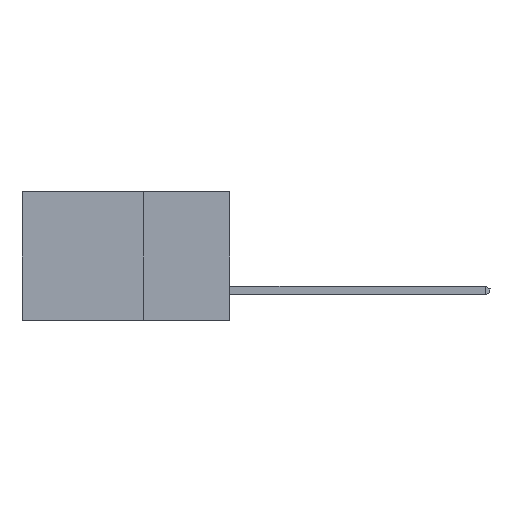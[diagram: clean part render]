
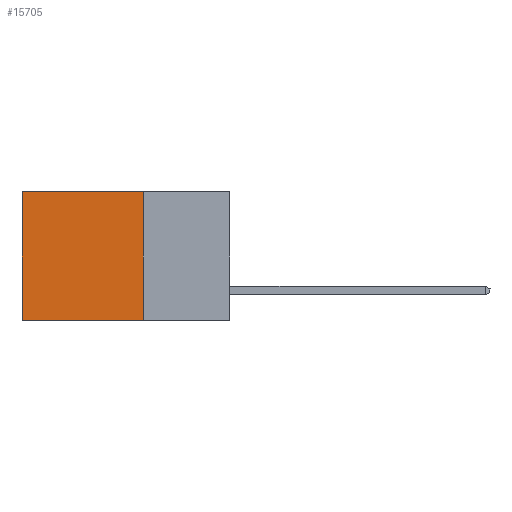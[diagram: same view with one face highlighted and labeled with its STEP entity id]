
A CAD part, left-side view. The second image highlights one B-rep face of the part: STEP entity #15705.
In plain terms, the highlighted planar face has unit normal (-1, 0, 0).
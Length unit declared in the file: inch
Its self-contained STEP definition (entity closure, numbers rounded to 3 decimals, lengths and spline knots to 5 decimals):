
#1093 = VERTEX_POINT ( 'NONE', #7252 ) ;
#1195 = DIRECTION ( 'NONE',  ( 0., 0., -1. ) ) ;
#1316 = ORIENTED_EDGE ( 'NONE', *, *, #8165, .T. ) ;
#1537 = AXIS2_PLACEMENT_3D ( 'NONE', #11090, #6801, #6607 ) ;
#2437 = ORIENTED_EDGE ( 'NONE', *, *, #10754, .F. ) ;
#2819 = EDGE_CURVE ( 'NONE', #3945, #1093, #11058, .T. ) ;
#3433 = LINE ( 'NONE', #9381, #17331 ) ;
#3897 = EDGE_LOOP ( 'NONE', ( #1316, #7428, #2437, #6747 ) ) ;
#3945 = VERTEX_POINT ( 'NONE', #3963 ) ;
#3952 = LINE ( 'NONE', #8041, #9803 ) ;
#3963 = CARTESIAN_POINT ( 'NONE',  ( 0.2615, 0.25, -0.37 ) ) ;
#5683 = CARTESIAN_POINT ( 'NONE',  ( 0.2615, 0.6, -0.37 ) ) ;
#6607 = DIRECTION ( 'NONE',  ( 0., 0., -1. ) ) ;
#6747 = ORIENTED_EDGE ( 'NONE', *, *, #13581, .T. ) ;
#6771 = DIRECTION ( 'NONE',  ( 0., 1., 0. ) ) ;
#6801 = DIRECTION ( 'NONE',  ( 1., 0., 0. ) ) ;
#7252 = CARTESIAN_POINT ( 'NONE',  ( 0.2615, 0.6, -0.37 ) ) ;
#7428 = ORIENTED_EDGE ( 'NONE', *, *, #2819, .F. ) ;
#7778 = VERTEX_POINT ( 'NONE', #10362 ) ;
#8041 = CARTESIAN_POINT ( 'NONE',  ( 0.2615, 0.25, -0.37 ) ) ;
#8165 = EDGE_CURVE ( 'NONE', #14528, #1093, #9878, .T. ) ;
#9051 = VECTOR ( 'NONE', #6771, 39.37008 ) ;
#9381 = CARTESIAN_POINT ( 'NONE',  ( 0.2615, 0.25, 0. ) ) ;
#9476 = VECTOR ( 'NONE', #1195, 39.37008 ) ;
#9803 = VECTOR ( 'NONE', #9891, 39.37008 ) ;
#9878 = LINE ( 'NONE', #5683, #9476 ) ;
#9891 = DIRECTION ( 'NONE',  ( 0., 0., -1. ) ) ;
#10362 = CARTESIAN_POINT ( 'NONE',  ( 0.2615, 0.25, 0. ) ) ;
#10754 = EDGE_CURVE ( 'NONE', #7778, #3945, #3952, .T. ) ;
#11058 = LINE ( 'NONE', #17271, #9051 ) ;
#11090 = CARTESIAN_POINT ( 'NONE',  ( 0.2615, 0.25, -0.37 ) ) ;
#11270 = PLANE ( 'NONE',  #1537 ) ;
#12619 = FACE_OUTER_BOUND ( 'NONE', #3897, .T. ) ;
#13581 = EDGE_CURVE ( 'NONE', #7778, #14528, #3433, .T. ) ;
#14528 = VERTEX_POINT ( 'NONE', #17016 ) ;
#15705 = ADVANCED_FACE ( 'NONE', ( #12619 ), #11270, .F. ) ;
#17016 = CARTESIAN_POINT ( 'NONE',  ( 0.2615, 0.6, 0. ) ) ;
#17271 = CARTESIAN_POINT ( 'NONE',  ( 0.2615, 0.25, -0.37 ) ) ;
#17331 = VECTOR ( 'NONE', #18317, 39.37008 ) ;
#18317 = DIRECTION ( 'NONE',  ( 0., 1., 0. ) ) ;
